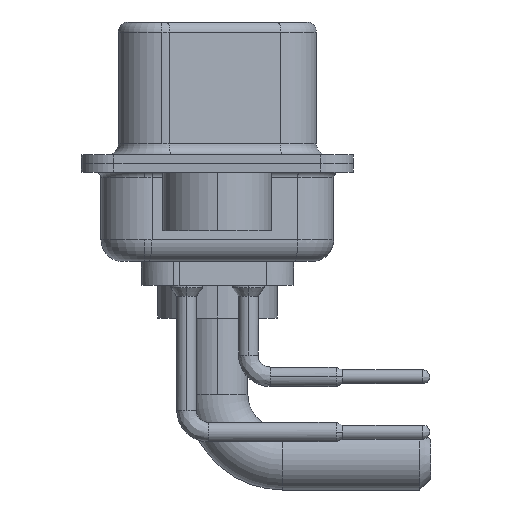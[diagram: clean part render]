
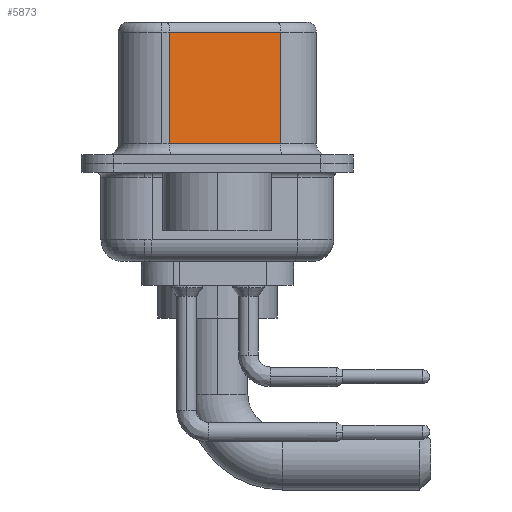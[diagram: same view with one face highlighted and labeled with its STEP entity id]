
A CAD part, left-side view. The second image highlights one B-rep face of the part: STEP entity #5873.
In plain terms, the highlighted planar face has unit normal (-0.985, -0.174, 0).
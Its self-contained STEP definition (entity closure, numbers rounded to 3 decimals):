
#979 = CARTESIAN_POINT ( 'NONE',  ( 4.58, -2.897, 6.02 ) ) ;
#1864 = CARTESIAN_POINT ( 'NONE',  ( 4.58, -2.897, 6.02 ) ) ;
#2469 = PLANE ( 'NONE',  #12817 ) ;
#2850 = DIRECTION ( 'NONE',  ( 0.174, -0.985, 0. ) ) ;
#4385 = CARTESIAN_POINT ( 'NONE',  ( 3.68, 2.203, 6.52 ) ) ;
#5024 = VECTOR ( 'NONE', #2850, 1000. ) ;
#5079 = LINE ( 'NONE', #21054, #21377 ) ;
#5738 = VERTEX_POINT ( 'NONE', #13514 ) ;
#5873 = ADVANCED_FACE ( 'NONE', ( #19917 ), #2469, .F. ) ;
#6629 = DIRECTION ( 'NONE',  ( -0.174, 0.985, 0. ) ) ;
#6900 = ORIENTED_EDGE ( 'NONE', *, *, #13273, .F. ) ;
#8308 = CARTESIAN_POINT ( 'NONE',  ( 4.58, -2.897, 0.9 ) ) ;
#8450 = EDGE_CURVE ( 'NONE', #5738, #25180, #19106, .T. ) ;
#10090 = DIRECTION ( 'NONE',  ( -0.174, 0.985, 0. ) ) ;
#10276 = ORIENTED_EDGE ( 'NONE', *, *, #8450, .T. ) ;
#11368 = CARTESIAN_POINT ( 'NONE',  ( 3.68, 2.203, 6.02 ) ) ;
#12246 = EDGE_CURVE ( 'NONE', #24446, #5738, #18665, .T. ) ;
#12817 = AXIS2_PLACEMENT_3D ( 'NONE', #18473, #22002, #10090 ) ;
#13273 = EDGE_CURVE ( 'NONE', #18696, #25180, #5079, .T. ) ;
#13514 = CARTESIAN_POINT ( 'NONE',  ( 3.68, 2.203, 0.9 ) ) ;
#15278 = EDGE_CURVE ( 'NONE', #18696, #24446, #18560, .T. ) ;
#16746 = VECTOR ( 'NONE', #18546, 1000. ) ;
#17013 = CARTESIAN_POINT ( 'NONE',  ( 4.58, -2.897, 0.9 ) ) ;
#17059 = EDGE_LOOP ( 'NONE', ( #6900, #25417, #17585, #10276 ) ) ;
#17585 = ORIENTED_EDGE ( 'NONE', *, *, #12246, .T. ) ;
#18473 = CARTESIAN_POINT ( 'NONE',  ( 4.58, -2.897, 6.52 ) ) ;
#18546 = DIRECTION ( 'NONE',  ( 0., 0., -1. ) ) ;
#18560 = LINE ( 'NONE', #979, #21374 ) ;
#18665 = LINE ( 'NONE', #4385, #16746 ) ;
#18696 = VERTEX_POINT ( 'NONE', #1864 ) ;
#19106 = LINE ( 'NONE', #17013, #5024 ) ;
#19917 = FACE_OUTER_BOUND ( 'NONE', #17059, .T. ) ;
#21054 = CARTESIAN_POINT ( 'NONE',  ( 4.58, -2.897, 6.52 ) ) ;
#21308 = DIRECTION ( 'NONE',  ( 0., 0., -1. ) ) ;
#21374 = VECTOR ( 'NONE', #6629, 1000. ) ;
#21377 = VECTOR ( 'NONE', #21308, 1000. ) ;
#22002 = DIRECTION ( 'NONE',  ( 0.985, 0.174, 0. ) ) ;
#24446 = VERTEX_POINT ( 'NONE', #11368 ) ;
#25180 = VERTEX_POINT ( 'NONE', #8308 ) ;
#25417 = ORIENTED_EDGE ( 'NONE', *, *, #15278, .T. ) ;
